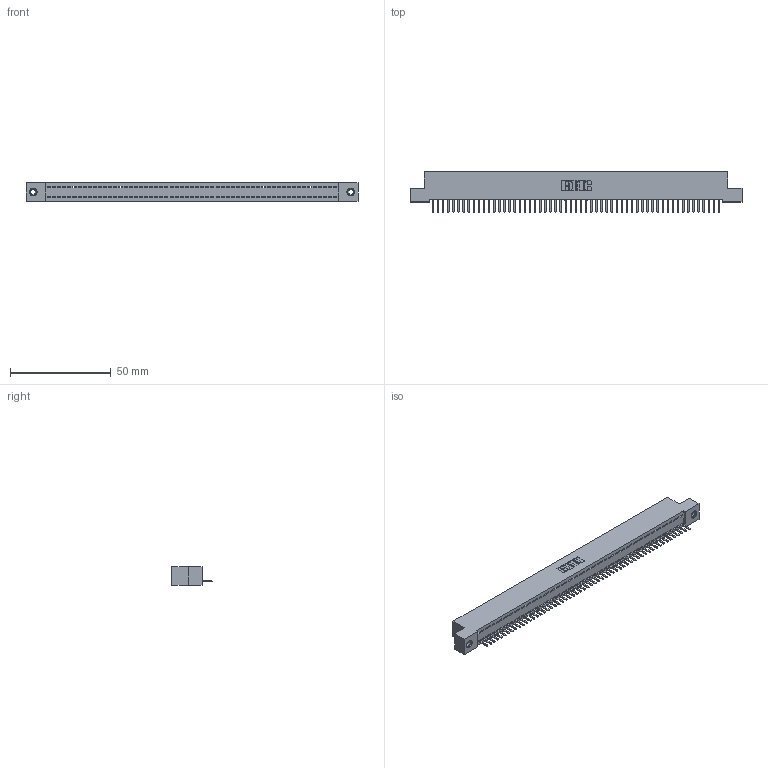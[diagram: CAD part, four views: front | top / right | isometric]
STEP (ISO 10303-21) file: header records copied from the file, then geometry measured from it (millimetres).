
FILE_DESCRIPTION (( 'STEP AP203' ), '1' );
FILE_NAME ('392-057-520-108.STEP', '2018-08-17T14:39:22', ( '' ), ( '' ), 'SwSTEP 2.0', 'SolidWorks 2016', '' );
FILE_SCHEMA (( 'CONFIG_CONTROL_DESIGN' ));
Length unit declared in the file: inch
Products named in the file (4): 392-057-520-108; 342 Part_TI; 345-292-001_345-293-120; 345-250-001_345-250-003-102
Assembly tree (60 placements, depth 2):
  392-057-520-108
    342 Part_TI
    345-292-001_345-293-120  x57
    345-250-001_345-250-003-102  x2
Bounding box: 165.1 x 20.02 x 9.4 mm (x, y, z)
Volume: 14361.6 mm3; surface area: 20862.8 mm2
Topology: 60 solids, 60 shells, 3704 faces, 10923 edges, 7122 vertices
Faces by surface type: plane 2606, cylinder 1082, cone 12, torus 4
Entity records: 34074 total; most frequent: CARTESIAN_POINT 5868, ORIENTED_EDGE 5842, DIRECTION 4941, EDGE_CURVE 2921, LINE 2769, VECTOR 2769, VERTEX_POINT 1940, AXIS2_PLACEMENT_3D 1086
